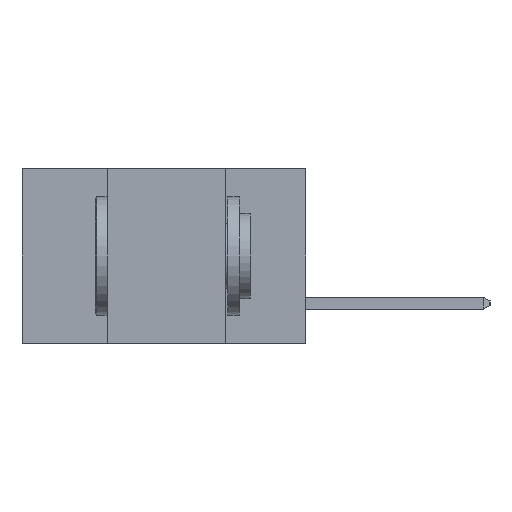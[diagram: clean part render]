
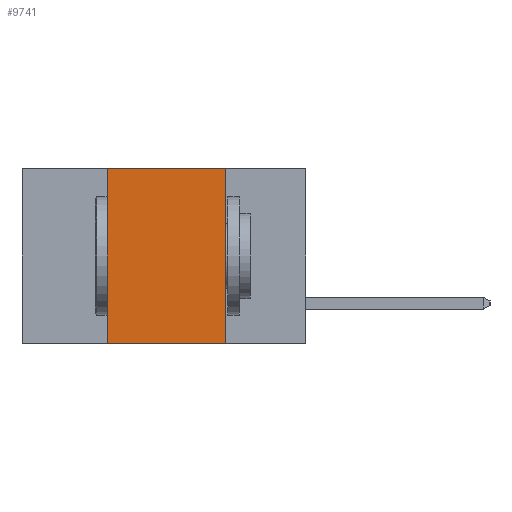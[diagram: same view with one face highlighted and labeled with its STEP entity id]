
A CAD part, left-side view. The second image highlights one B-rep face of the part: STEP entity #9741.
In plain terms, the highlighted planar face has unit normal (-1, 0, 0).
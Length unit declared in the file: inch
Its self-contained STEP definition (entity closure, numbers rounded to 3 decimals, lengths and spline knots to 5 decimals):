
#150 = CARTESIAN_POINT ( 'NONE',  ( 0., 0.42, 0. ) ) ;
#179 = VERTEX_POINT ( 'NONE', #7206 ) ;
#524 = LINE ( 'NONE', #896, #5088 ) ;
#896 = CARTESIAN_POINT ( 'NONE',  ( 0., 0.42, -0.37 ) ) ;
#898 = CARTESIAN_POINT ( 'NONE',  ( 0., 0.6, -0.37 ) ) ;
#1029 = DIRECTION ( 'NONE',  ( 0., 0., 1. ) ) ;
#1302 = LINE ( 'NONE', #898, #10406 ) ;
#2303 = EDGE_CURVE ( 'NONE', #179, #9029, #9504, .T. ) ;
#2725 = DIRECTION ( 'NONE',  ( 0., -1., 0. ) ) ;
#2937 = AXIS2_PLACEMENT_3D ( 'NONE', #7027, #10494, #5278 ) ;
#3156 = ORIENTED_EDGE ( 'NONE', *, *, #4794, .F. ) ;
#4061 = EDGE_LOOP ( 'NONE', ( #7751, #7886, #3156, #7537 ) ) ;
#4413 = PLANE ( 'NONE',  #2937 ) ;
#4794 = EDGE_CURVE ( 'NONE', #6026, #9320, #524, .T. ) ;
#4871 = VECTOR ( 'NONE', #7289, 39.37008 ) ;
#5088 = VECTOR ( 'NONE', #1029, 39.37008 ) ;
#5278 = DIRECTION ( 'NONE',  ( 0., 0., -1. ) ) ;
#6026 = VERTEX_POINT ( 'NONE', #6973 ) ;
#6973 = CARTESIAN_POINT ( 'NONE',  ( 0., 0.42, -0.37 ) ) ;
#7027 = CARTESIAN_POINT ( 'NONE',  ( 0., 0.6, 0. ) ) ;
#7185 = CARTESIAN_POINT ( 'NONE',  ( 0., 0.6, 0. ) ) ;
#7206 = CARTESIAN_POINT ( 'NONE',  ( 0., 0.17, 0. ) ) ;
#7243 = VECTOR ( 'NONE', #2725, 39.37008 ) ;
#7276 = FACE_OUTER_BOUND ( 'NONE', #4061, .T. ) ;
#7280 = CARTESIAN_POINT ( 'NONE',  ( 0., 0.17, -0.37 ) ) ;
#7289 = DIRECTION ( 'NONE',  ( 0., 0., -1. ) ) ;
#7504 = LINE ( 'NONE', #7185, #7243 ) ;
#7537 = ORIENTED_EDGE ( 'NONE', *, *, #9158, .T. ) ;
#7751 = ORIENTED_EDGE ( 'NONE', *, *, #2303, .F. ) ;
#7886 = ORIENTED_EDGE ( 'NONE', *, *, #11111, .F. ) ;
#8708 = CARTESIAN_POINT ( 'NONE',  ( 0., 0.17, -0.37 ) ) ;
#8928 = DIRECTION ( 'NONE',  ( 0., -1., 0. ) ) ;
#9029 = VERTEX_POINT ( 'NONE', #8708 ) ;
#9158 = EDGE_CURVE ( 'NONE', #6026, #9029, #1302, .T. ) ;
#9320 = VERTEX_POINT ( 'NONE', #150 ) ;
#9504 = LINE ( 'NONE', #7280, #4871 ) ;
#9741 = ADVANCED_FACE ( 'NONE', ( #7276 ), #4413, .F. ) ;
#10406 = VECTOR ( 'NONE', #8928, 39.37008 ) ;
#10494 = DIRECTION ( 'NONE',  ( 1., 0., 0. ) ) ;
#11111 = EDGE_CURVE ( 'NONE', #9320, #179, #7504, .T. ) ;
